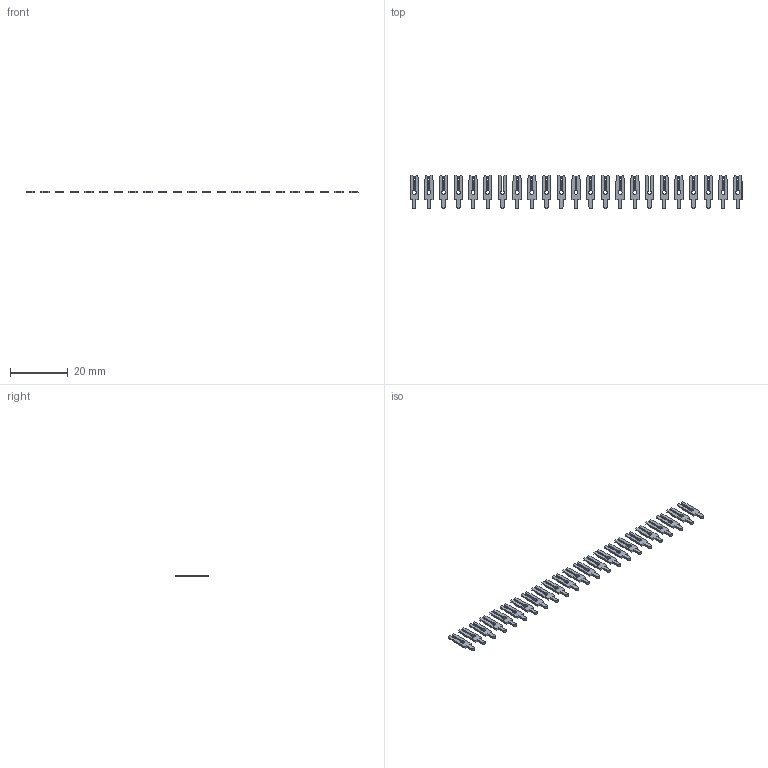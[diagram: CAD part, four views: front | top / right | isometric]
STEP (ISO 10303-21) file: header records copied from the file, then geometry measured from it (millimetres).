
FILE_DESCRIPTION (( 'STEP AP203' ), '1' );
FILE_NAME ('103-023-250-200.STEP', '2020-04-09T20:37:47', ( '' ), ( '' ), 'SwSTEP 2.0', 'SolidWorks 2016', '' );
FILE_SCHEMA (( 'CONFIG_CONTROL_DESIGN' ));
Length unit declared in the file: inch
Products named in the file (2): 103-023-250-200; 100-290-001_100-290-250
Assembly tree (23 placements, depth 2):
  103-023-250-200
    100-290-001_100-290-250  x23
Bounding box: 114.68 x 11.48 x 0.66 mm (x, y, z)
Volume: 358.9 mm3; surface area: 1687 mm2
Topology: 23 solids, 23 shells, 552 faces, 1518 edges, 1012 vertices
Faces by surface type: plane 460, cylinder 92
Entity records: 1662 total; most frequent: CARTESIAN_POINT 172, DIRECTION 170, ORIENTED_EDGE 132, EDGE_CURVE 66, AXIS2_PLACEMENT_3D 58, COORDINATED_UNIVERSAL_TIME_OFFSET 56, LOCAL_TIME 56, DATE_AND_TIME 56
